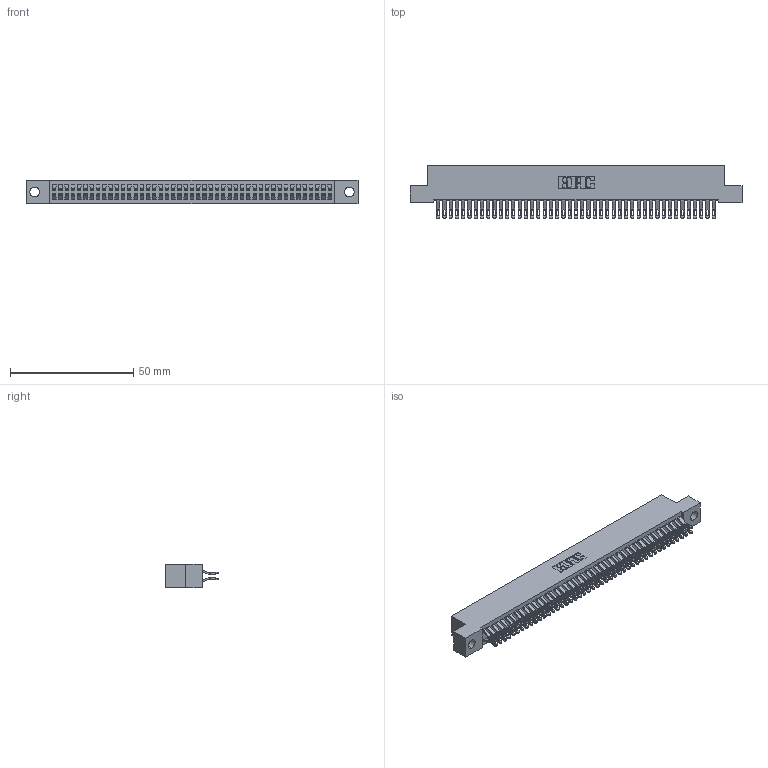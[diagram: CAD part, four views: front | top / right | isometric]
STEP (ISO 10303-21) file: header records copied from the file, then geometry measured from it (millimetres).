
FILE_DESCRIPTION (( 'STEP AP203' ), '1' );
FILE_NAME ('392-090-555-204.STEP', '2019-10-09T18:33:18', ( '' ), ( '' ), 'SwSTEP 2.0', 'SolidWorks 2016', '' );
FILE_SCHEMA (( 'CONFIG_CONTROL_DESIGN' ));
Length unit declared in the file: inch
Products named in the file (3): 345-292-001_555 Tail; 392-090-555-204; 342 Part_.156 TH
Assembly tree (91 placements, depth 2):
  392-090-555-204
    342 Part_.156 TH
    345-292-001_555 Tail  x90
Bounding box: 134.62 x 21.47 x 9.4 mm (x, y, z)
Volume: 12272.9 mm3; surface area: 20746.1 mm2
Topology: 91 solids, 91 shells, 5330 faces, 16769 edges, 11178 vertices
Faces by surface type: plane 3126, cylinder 2204
Entity records: 28759 total; most frequent: CARTESIAN_POINT 4796, ORIENTED_EDGE 4702, DIRECTION 4063, EDGE_CURVE 2351, LINE 2203, VECTOR 2203, VERTEX_POINT 1566, AXIS2_PLACEMENT_3D 930
